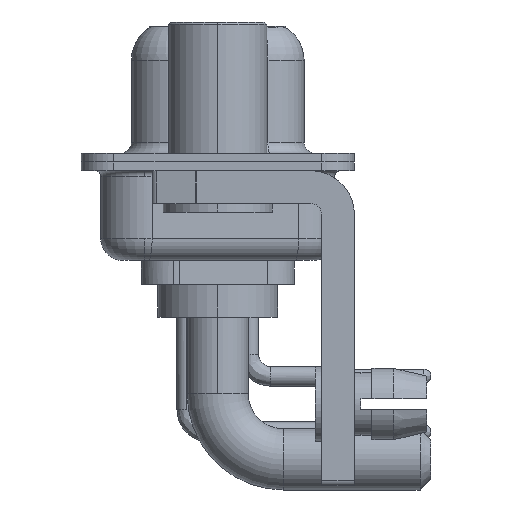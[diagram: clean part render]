
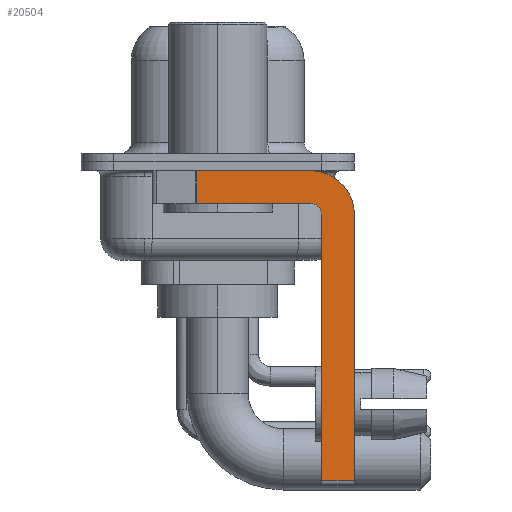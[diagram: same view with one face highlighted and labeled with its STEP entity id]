
A CAD part, left-side view. The second image highlights one B-rep face of the part: STEP entity #20504.
In plain terms, the highlighted planar face has unit normal (-1, 0, 0).
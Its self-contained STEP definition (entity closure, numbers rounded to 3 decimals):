
#71 = VERTEX_POINT ( 'NONE', #5071 ) ;
#289 = CARTESIAN_POINT ( 'NONE',  ( -2.9, 0.978, -1.9 ) ) ;
#975 = ORIENTED_EDGE ( 'NONE', *, *, #8794, .F. ) ;
#1184 = CARTESIAN_POINT ( 'NONE',  ( -2.9, -4.75, -14.8 ) ) ;
#1635 = CARTESIAN_POINT ( 'NONE',  ( -2.9, -4.25, -2.4 ) ) ;
#2078 = CARTESIAN_POINT ( 'NONE',  ( -2.9, -4.75, -2.4 ) ) ;
#2786 = CARTESIAN_POINT ( 'NONE',  ( -2.9, -4.25, -2.4 ) ) ;
#2936 = CARTESIAN_POINT ( 'NONE',  ( -2.9, -4.75, -14.55 ) ) ;
#3537 = EDGE_CURVE ( 'NONE', #22026, #16284, #23133, .T. ) ;
#4034 = VECTOR ( 'NONE', #8585, 1000. ) ;
#4196 = LINE ( 'NONE', #12906, #18731 ) ;
#4488 = CIRCLE ( 'NONE', #21004, 0.5 ) ;
#4684 = VECTOR ( 'NONE', #18158, 1000. ) ;
#4707 = CARTESIAN_POINT ( 'NONE',  ( -2.9, -4.25, -0.4 ) ) ;
#5007 = CARTESIAN_POINT ( 'NONE',  ( -2.9, -6.25, -2.4 ) ) ;
#5071 = CARTESIAN_POINT ( 'NONE',  ( -2.9, -6.25, -14.55 ) ) ;
#5850 = VECTOR ( 'NONE', #12271, 1000. ) ;
#5972 = EDGE_CURVE ( 'NONE', #15685, #71, #6754, .T. ) ;
#6255 = EDGE_CURVE ( 'NONE', #15685, #7861, #10209, .T. ) ;
#6577 = EDGE_CURVE ( 'NONE', #16284, #71, #4196, .T. ) ;
#6754 = LINE ( 'NONE', #23170, #5850 ) ;
#6881 = VERTEX_POINT ( 'NONE', #21512 ) ;
#7147 = DIRECTION ( 'NONE',  ( 1., 0., 0. ) ) ;
#7390 = AXIS2_PLACEMENT_3D ( 'NONE', #1635, #7147, #12433 ) ;
#7861 = VERTEX_POINT ( 'NONE', #2078 ) ;
#7886 = DIRECTION ( 'NONE',  ( 1., 0., 0. ) ) ;
#7970 = LINE ( 'NONE', #16999, #21899 ) ;
#7992 = CARTESIAN_POINT ( 'NONE',  ( -2.9, -4.25, -2.4 ) ) ;
#8585 = DIRECTION ( 'NONE',  ( 0., 0., 1. ) ) ;
#8743 = VERTEX_POINT ( 'NONE', #16890 ) ;
#8794 = EDGE_CURVE ( 'NONE', #8743, #22380, #7970, .T. ) ;
#9401 = DIRECTION ( 'NONE',  ( 0., 0., -1. ) ) ;
#9449 = ORIENTED_EDGE ( 'NONE', *, *, #17402, .F. ) ;
#10209 = LINE ( 'NONE', #1184, #4034 ) ;
#11166 = CARTESIAN_POINT ( 'NONE',  ( -2.9, 0.978, -1.9 ) ) ;
#11398 = ORIENTED_EDGE ( 'NONE', *, *, #18004, .T. ) ;
#12271 = DIRECTION ( 'NONE',  ( 0., -1., 0. ) ) ;
#12433 = DIRECTION ( 'NONE',  ( 0., 0., -1. ) ) ;
#12906 = CARTESIAN_POINT ( 'NONE',  ( -2.9, -6.25, -2.4 ) ) ;
#13075 = ORIENTED_EDGE ( 'NONE', *, *, #6577, .F. ) ;
#13090 = EDGE_LOOP ( 'NONE', ( #21441, #11398, #975, #9449, #20095, #17492, #13075, #19727 ) ) ;
#13243 = DIRECTION ( 'NONE',  ( 0., 0., -1. ) ) ;
#13275 = PLANE ( 'NONE',  #20028 ) ;
#14603 = DIRECTION ( 'NONE',  ( 0., 0., -1. ) ) ;
#14991 = DIRECTION ( 'NONE',  ( -1., 0., 0. ) ) ;
#15685 = VERTEX_POINT ( 'NONE', #2936 ) ;
#16284 = VERTEX_POINT ( 'NONE', #5007 ) ;
#16890 = CARTESIAN_POINT ( 'NONE',  ( -2.9, -4.25, -1.9 ) ) ;
#16999 = CARTESIAN_POINT ( 'NONE',  ( -2.9, -4.25, -1.9 ) ) ;
#17108 = DIRECTION ( 'NONE',  ( 0., 0., 1. ) ) ;
#17402 = EDGE_CURVE ( 'NONE', #7861, #8743, #4488, .T. ) ;
#17492 = ORIENTED_EDGE ( 'NONE', *, *, #5972, .T. ) ;
#18004 = EDGE_CURVE ( 'NONE', #6881, #22380, #22976, .T. ) ;
#18158 = DIRECTION ( 'NONE',  ( 0., -1., 0. ) ) ;
#18282 = CARTESIAN_POINT ( 'NONE',  ( -2.9, 3., -0.4 ) ) ;
#18430 = DIRECTION ( 'NONE',  ( 0., 1., 0. ) ) ;
#18731 = VECTOR ( 'NONE', #13243, 1000. ) ;
#19528 = VECTOR ( 'NONE', #14603, 1000. ) ;
#19727 = ORIENTED_EDGE ( 'NONE', *, *, #3537, .F. ) ;
#20028 = AXIS2_PLACEMENT_3D ( 'NONE', #7992, #7886, #9401 ) ;
#20095 = ORIENTED_EDGE ( 'NONE', *, *, #6255, .F. ) ;
#20160 = LINE ( 'NONE', #18282, #4684 ) ;
#20504 = ADVANCED_FACE ( 'NONE', ( #22306 ), #13275, .F. ) ;
#21004 = AXIS2_PLACEMENT_3D ( 'NONE', #2786, #14991, #17108 ) ;
#21441 = ORIENTED_EDGE ( 'NONE', *, *, #21522, .F. ) ;
#21512 = CARTESIAN_POINT ( 'NONE',  ( -2.9, 0.978, -0.4 ) ) ;
#21522 = EDGE_CURVE ( 'NONE', #6881, #22026, #20160, .T. ) ;
#21899 = VECTOR ( 'NONE', #18430, 1000. ) ;
#22026 = VERTEX_POINT ( 'NONE', #4707 ) ;
#22306 = FACE_OUTER_BOUND ( 'NONE', #13090, .T. ) ;
#22380 = VERTEX_POINT ( 'NONE', #11166 ) ;
#22976 = LINE ( 'NONE', #289, #19528 ) ;
#23133 = CIRCLE ( 'NONE', #7390, 2. ) ;
#23170 = CARTESIAN_POINT ( 'NONE',  ( -2.9, -4.25, -14.55 ) ) ;
